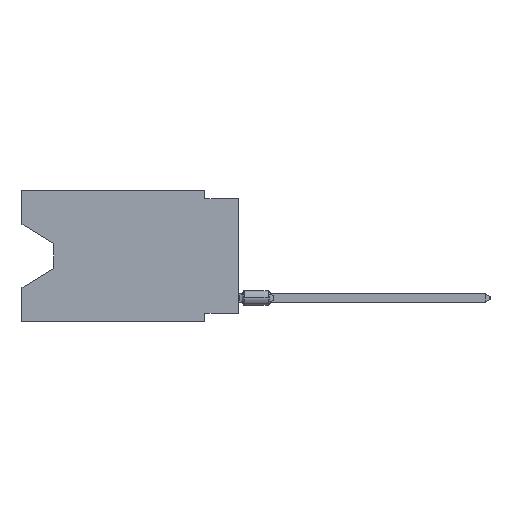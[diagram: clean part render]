
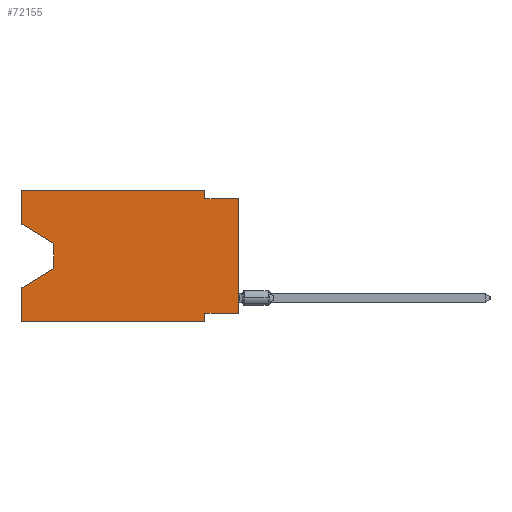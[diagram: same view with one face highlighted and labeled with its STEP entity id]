
A CAD part, left-side view. The second image highlights one B-rep face of the part: STEP entity #72155.
In plain terms, the highlighted planar face has unit normal (-1, 0, 0).
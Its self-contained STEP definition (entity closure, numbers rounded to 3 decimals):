
#754 = ORIENTED_EDGE ( 'NONE', *, *, #2741, .T. ) ;
#1153 = LINE ( 'NONE', #15999, #73992 ) ;
#1295 = ORIENTED_EDGE ( 'NONE', *, *, #49821, .F. ) ;
#1603 = LINE ( 'NONE', #21574, #59340 ) ;
#1743 = CARTESIAN_POINT ( 'NONE',  ( 0., 2.54, -9.906 ) ) ;
#1816 = VECTOR ( 'NONE', #64021, 1000. ) ;
#2032 = LINE ( 'NONE', #52616, #34939 ) ;
#2741 = EDGE_CURVE ( 'NONE', #43636, #30818, #1153, .T. ) ;
#2776 = CARTESIAN_POINT ( 'NONE',  ( 0., 2.54, -0.635 ) ) ;
#3335 = DIRECTION ( 'NONE',  ( 0., 0., 1. ) ) ;
#5441 = VECTOR ( 'NONE', #45566, 1000. ) ;
#5937 = LINE ( 'NONE', #31866, #40443 ) ;
#6261 = CARTESIAN_POINT ( 'NONE',  ( 0., 16.383, 0. ) ) ;
#6519 = VECTOR ( 'NONE', #81154, 1000. ) ;
#9034 = VERTEX_POINT ( 'NONE', #1743 ) ;
#9343 = EDGE_CURVE ( 'NONE', #15039, #39425, #5937, .T. ) ;
#11803 = PLANE ( 'NONE',  #49903 ) ;
#13633 = CARTESIAN_POINT ( 'NONE',  ( 0., 2.54, -9.271 ) ) ;
#13712 = CARTESIAN_POINT ( 'NONE',  ( 0., 16.383, -9.906 ) ) ;
#15039 = VERTEX_POINT ( 'NONE', #71241 ) ;
#15999 = CARTESIAN_POINT ( 'NONE',  ( 0., 13.97, -5.893 ) ) ;
#19231 = EDGE_LOOP ( 'NONE', ( #29708, #22306, #754, #45092, #71935, #25357, #1295, #52773, #66869, #64108, #33345, #49847 ) ) ;
#21173 = LINE ( 'NONE', #40730, #69483 ) ;
#21226 = EDGE_CURVE ( 'NONE', #37371, #9034, #61059, .T. ) ;
#21574 = CARTESIAN_POINT ( 'NONE',  ( 0., 13.97, -4.013 ) ) ;
#22306 = ORIENTED_EDGE ( 'NONE', *, *, #47827, .T. ) ;
#25357 = ORIENTED_EDGE ( 'NONE', *, *, #21226, .F. ) ;
#26460 = CARTESIAN_POINT ( 'NONE',  ( 0., 13.97, -5.893 ) ) ;
#27313 = CARTESIAN_POINT ( 'NONE',  ( 0., 0., -0.635 ) ) ;
#28567 = VERTEX_POINT ( 'NONE', #13712 ) ;
#29708 = ORIENTED_EDGE ( 'NONE', *, *, #39196, .T. ) ;
#30446 = VERTEX_POINT ( 'NONE', #27313 ) ;
#30818 = VERTEX_POINT ( 'NONE', #64287 ) ;
#30903 = CARTESIAN_POINT ( 'NONE',  ( 0., 13.97, -4.013 ) ) ;
#31004 = VECTOR ( 'NONE', #36610, 1000. ) ;
#31668 = VECTOR ( 'NONE', #75114, 1000. ) ;
#31866 = CARTESIAN_POINT ( 'NONE',  ( 0., 2.54, 0. ) ) ;
#33345 = ORIENTED_EDGE ( 'NONE', *, *, #39173, .F. ) ;
#34939 = VECTOR ( 'NONE', #40281, 1000. ) ;
#35219 = VERTEX_POINT ( 'NONE', #56373 ) ;
#36610 = DIRECTION ( 'NONE',  ( 0., 1., 0. ) ) ;
#37170 = VECTOR ( 'NONE', #54689, 1000. ) ;
#37371 = VERTEX_POINT ( 'NONE', #13633 ) ;
#37734 = DIRECTION ( 'NONE',  ( 1., 0., 0. ) ) ;
#39173 = EDGE_CURVE ( 'NONE', #35219, #15039, #44083, .T. ) ;
#39179 = CARTESIAN_POINT ( 'NONE',  ( 0., 0., 0. ) ) ;
#39196 = EDGE_CURVE ( 'NONE', #51665, #44132, #83154, .T. ) ;
#39425 = VERTEX_POINT ( 'NONE', #2776 ) ;
#40281 = DIRECTION ( 'NONE',  ( 0., 0., 1. ) ) ;
#40443 = VECTOR ( 'NONE', #57787, 1000. ) ;
#40635 = CARTESIAN_POINT ( 'NONE',  ( 0., 0., -0.635 ) ) ;
#40730 = CARTESIAN_POINT ( 'NONE',  ( 0., 16.383, 0. ) ) ;
#41126 = DIRECTION ( 'NONE',  ( 0., 0., -1. ) ) ;
#43636 = VERTEX_POINT ( 'NONE', #26460 ) ;
#44083 = LINE ( 'NONE', #81902, #1816 ) ;
#44132 = VERTEX_POINT ( 'NONE', #30903 ) ;
#45092 = ORIENTED_EDGE ( 'NONE', *, *, #63005, .F. ) ;
#45566 = DIRECTION ( 'NONE',  ( 0., 0., 1. ) ) ;
#47827 = EDGE_CURVE ( 'NONE', #44132, #43636, #1603, .T. ) ;
#48109 = CARTESIAN_POINT ( 'NONE',  ( 0., 0., -9.271 ) ) ;
#49821 = EDGE_CURVE ( 'NONE', #84023, #37371, #75291, .T. ) ;
#49847 = ORIENTED_EDGE ( 'NONE', *, *, #56130, .F. ) ;
#49903 = AXIS2_PLACEMENT_3D ( 'NONE', #6261, #37734, #77635 ) ;
#51610 = EDGE_CURVE ( 'NONE', #39425, #30446, #64868, .T. ) ;
#51665 = VERTEX_POINT ( 'NONE', #73331 ) ;
#52616 = CARTESIAN_POINT ( 'NONE',  ( 0., 16.383, 0. ) ) ;
#52773 = ORIENTED_EDGE ( 'NONE', *, *, #53626, .T. ) ;
#53626 = EDGE_CURVE ( 'NONE', #84023, #30446, #58307, .T. ) ;
#54689 = DIRECTION ( 'NONE',  ( 0., 0., -1. ) ) ;
#56130 = EDGE_CURVE ( 'NONE', #51665, #35219, #21173, .T. ) ;
#56373 = CARTESIAN_POINT ( 'NONE',  ( 0., 16.383, 0. ) ) ;
#57787 = DIRECTION ( 'NONE',  ( 0., 0., -1. ) ) ;
#58307 = LINE ( 'NONE', #39179, #5441 ) ;
#59340 = VECTOR ( 'NONE', #41126, 1000. ) ;
#60215 = CARTESIAN_POINT ( 'NONE',  ( 0., 2.54, -9.906 ) ) ;
#61059 = LINE ( 'NONE', #60215, #37170 ) ;
#63005 = EDGE_CURVE ( 'NONE', #28567, #30818, #2032, .T. ) ;
#64021 = DIRECTION ( 'NONE',  ( 0., -1., 0. ) ) ;
#64108 = ORIENTED_EDGE ( 'NONE', *, *, #9343, .F. ) ;
#64287 = CARTESIAN_POINT ( 'NONE',  ( 0., 16.383, -7.36 ) ) ;
#64868 = LINE ( 'NONE', #40635, #67614 ) ;
#66869 = ORIENTED_EDGE ( 'NONE', *, *, #51610, .F. ) ;
#67614 = VECTOR ( 'NONE', #72916, 1000. ) ;
#69136 = CARTESIAN_POINT ( 'NONE',  ( 0., 16.383, -2.546 ) ) ;
#69483 = VECTOR ( 'NONE', #3335, 1000. ) ;
#71241 = CARTESIAN_POINT ( 'NONE',  ( 0., 2.54, 0. ) ) ;
#71935 = ORIENTED_EDGE ( 'NONE', *, *, #77583, .T. ) ;
#72155 = ADVANCED_FACE ( 'NONE', ( #83611 ), #11803, .F. ) ;
#72348 = CARTESIAN_POINT ( 'NONE',  ( 0., 16.383, -9.906 ) ) ;
#72775 = LINE ( 'NONE', #72348, #6519 ) ;
#72916 = DIRECTION ( 'NONE',  ( 0., -1., 0. ) ) ;
#73331 = CARTESIAN_POINT ( 'NONE',  ( 0., 16.383, -2.546 ) ) ;
#73372 = DIRECTION ( 'NONE',  ( 0., 0.855, -0.519 ) ) ;
#73992 = VECTOR ( 'NONE', #73372, 1000. ) ;
#75114 = DIRECTION ( 'NONE',  ( 0., -0.855, -0.519 ) ) ;
#75291 = LINE ( 'NONE', #48109, #31004 ) ;
#77583 = EDGE_CURVE ( 'NONE', #28567, #9034, #72775, .T. ) ;
#77635 = DIRECTION ( 'NONE',  ( 0., 0., -1. ) ) ;
#79390 = CARTESIAN_POINT ( 'NONE',  ( 0., 0., -9.271 ) ) ;
#81154 = DIRECTION ( 'NONE',  ( 0., -1., 0. ) ) ;
#81902 = CARTESIAN_POINT ( 'NONE',  ( 0., 16.383, 0. ) ) ;
#83154 = LINE ( 'NONE', #69136, #31668 ) ;
#83611 = FACE_OUTER_BOUND ( 'NONE', #19231, .T. ) ;
#84023 = VERTEX_POINT ( 'NONE', #79390 ) ;
